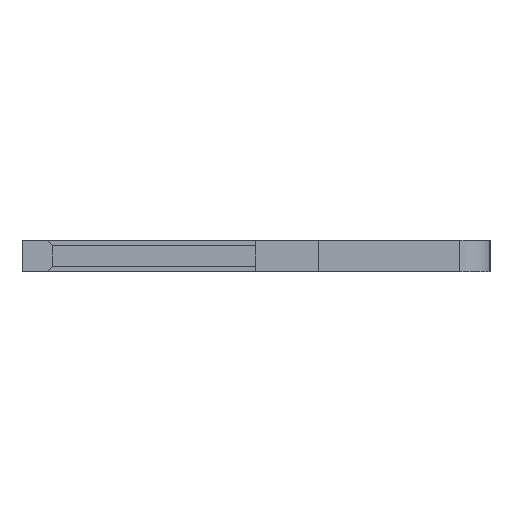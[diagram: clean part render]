
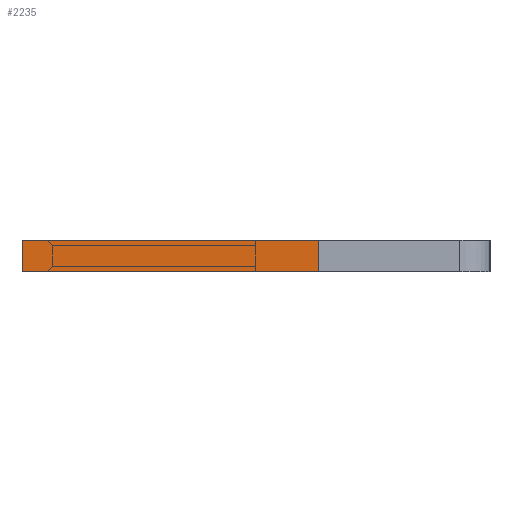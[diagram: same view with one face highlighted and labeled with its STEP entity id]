
A CAD part, left-side view. The second image highlights one B-rep face of the part: STEP entity #2235.
In plain terms, the highlighted face is planar.
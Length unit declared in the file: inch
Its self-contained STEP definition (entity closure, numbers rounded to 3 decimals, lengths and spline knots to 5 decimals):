
#4 = EDGE_CURVE ( 'NONE', #1515, #3354, #3146, .T. ) ;
#92 = CARTESIAN_POINT ( 'NONE',  ( 0.01, -0.04, -0.04 ) ) ;
#155 = CARTESIAN_POINT ( 'NONE',  ( -0.01, -0.04, -0.04 ) ) ;
#158 = VERTEX_POINT ( 'NONE', #2877 ) ;
#161 = AXIS2_PLACEMENT_3D ( 'NONE', #590, #924, #1805 ) ;
#261 = CARTESIAN_POINT ( 'NONE',  ( -0.01, 0.15, -0.04 ) ) ;
#390 = CARTESIAN_POINT ( 'NONE',  ( 0.01, -0.04, -0.04 ) ) ;
#590 = CARTESIAN_POINT ( 'NONE',  ( 0.01, 0.15, -0.04 ) ) ;
#614 = DIRECTION ( 'NONE',  ( 0., 1., 0. ) ) ;
#790 = DIRECTION ( 'NONE',  ( 0., 1., 0. ) ) ;
#850 = VECTOR ( 'NONE', #1666, 39.37008 ) ;
#894 = FACE_OUTER_BOUND ( 'NONE', #3637, .T. ) ;
#924 = DIRECTION ( 'NONE',  ( 0., 0., 1. ) ) ;
#1005 = CARTESIAN_POINT ( 'NONE',  ( 0.01, 0.15, -0.04 ) ) ;
#1008 = EDGE_CURVE ( 'NONE', #3983, #1515, #2068, .T. ) ;
#1110 = CARTESIAN_POINT ( 'NONE',  ( 0.01, 0.15, -0.04 ) ) ;
#1224 = LINE ( 'NONE', #1005, #1373 ) ;
#1373 = VECTOR ( 'NONE', #790, 39.37008 ) ;
#1480 = PLANE ( 'NONE',  #161 ) ;
#1515 = VERTEX_POINT ( 'NONE', #155 ) ;
#1666 = DIRECTION ( 'NONE',  ( -1., 0., 0. ) ) ;
#1805 = DIRECTION ( 'NONE',  ( 1., 0., 0. ) ) ;
#2068 = LINE ( 'NONE', #390, #850 ) ;
#2100 = ORIENTED_EDGE ( 'NONE', *, *, #3846, .F. ) ;
#2157 = EDGE_CURVE ( 'NONE', #158, #3354, #2275, .T. ) ;
#2167 = VECTOR ( 'NONE', #3638, 39.37008 ) ;
#2235 = ADVANCED_FACE ( 'NONE', ( #894 ), #1480, .F. ) ;
#2275 = LINE ( 'NONE', #1110, #2167 ) ;
#2448 = ORIENTED_EDGE ( 'NONE', *, *, #4, .T. ) ;
#2877 = CARTESIAN_POINT ( 'NONE',  ( 0.01, 0.15, -0.04 ) ) ;
#3146 = LINE ( 'NONE', #261, #3581 ) ;
#3149 = CARTESIAN_POINT ( 'NONE',  ( -0.01, 0.15, -0.04 ) ) ;
#3153 = ORIENTED_EDGE ( 'NONE', *, *, #2157, .F. ) ;
#3354 = VERTEX_POINT ( 'NONE', #3149 ) ;
#3454 = ORIENTED_EDGE ( 'NONE', *, *, #1008, .T. ) ;
#3581 = VECTOR ( 'NONE', #614, 39.37008 ) ;
#3637 = EDGE_LOOP ( 'NONE', ( #2448, #3153, #2100, #3454 ) ) ;
#3638 = DIRECTION ( 'NONE',  ( -1., 0., 0. ) ) ;
#3846 = EDGE_CURVE ( 'NONE', #3983, #158, #1224, .T. ) ;
#3983 = VERTEX_POINT ( 'NONE', #92 ) ;
